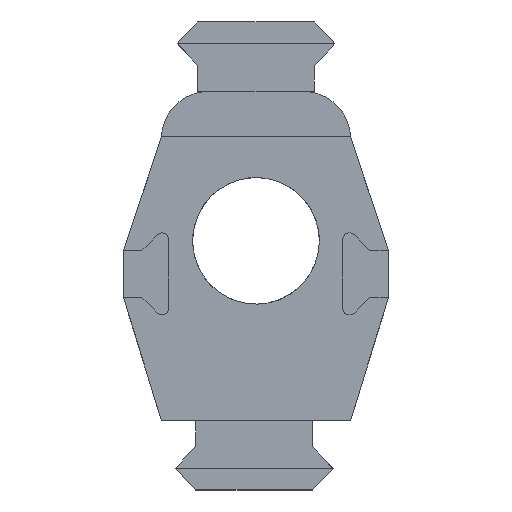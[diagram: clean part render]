
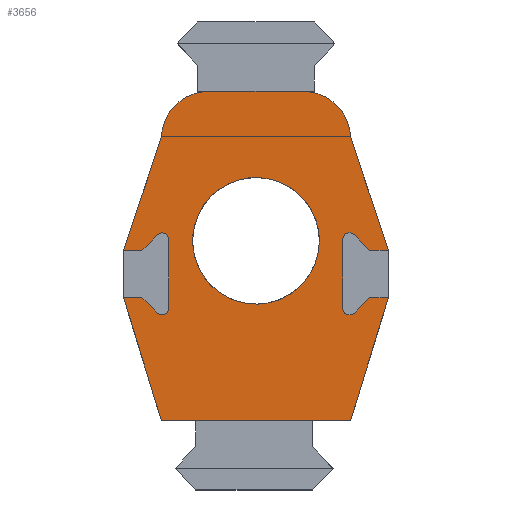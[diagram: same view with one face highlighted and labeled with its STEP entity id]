
A CAD part, front view. The second image highlights one B-rep face of the part: STEP entity #3656.
In plain terms, the highlighted planar face has unit normal (0, -1, 0).
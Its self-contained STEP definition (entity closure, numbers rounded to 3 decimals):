
#32=FACE_BOUND('',#323,.T.);
#36=ELLIPSE('',#3889,3.676,2.54);
#37=ELLIPSE('',#3892,3.676,2.54);
#56=CIRCLE('',#3868,0.889);
#58=CIRCLE('',#3872,0.889);
#60=CIRCLE('',#3878,0.889);
#62=CIRCLE('',#3882,0.889);
#64=CIRCLE('',#3890,6.35);
#65=CIRCLE('',#3891,6.35);
#66=CIRCLE('',#3893,8.5);
#67=CIRCLE('',#3894,8.5);
#117=FACE_OUTER_BOUND('',#322,.T.);
#322=EDGE_LOOP('',(#2455,#2456,#2457,#2458,#2459,#2460,#2461,#2462,#2463,
#2464,#2465,#2466,#2467,#2468,#2469,#2470,#2471,#2472,#2473,#2474,#2475,
#2476,#2477,#2478));
#323=EDGE_LOOP('',(#2479,#2480));
#515=LINE('',#5106,#1007);
#519=LINE('',#5115,#1011);
#523=LINE('',#5123,#1015);
#527=LINE('',#5135,#1019);
#531=LINE('',#5146,#1023);
#534=LINE('',#5153,#1026);
#539=LINE('',#5167,#1031);
#543=LINE('',#5179,#1035);
#546=LINE('',#5185,#1038);
#549=LINE('',#5191,#1041);
#554=LINE('',#5203,#1046);
#555=LINE('',#5205,#1047);
#556=LINE('',#5209,#1048);
#557=LINE('',#5212,#1049);
#558=LINE('',#5214,#1050);
#559=LINE('',#5217,#1051);
#1007=VECTOR('',#4116,10.);
#1011=VECTOR('',#4122,10.);
#1015=VECTOR('',#4128,10.);
#1019=VECTOR('',#4140,10.);
#1023=VECTOR('',#4152,10.);
#1026=VECTOR('',#4159,10.);
#1031=VECTOR('',#4172,10.);
#1035=VECTOR('',#4184,10.);
#1038=VECTOR('',#4189,10.);
#1041=VECTOR('',#4194,10.);
#1046=VECTOR('',#4205,10.);
#1047=VECTOR('',#4206,10.);
#1048=VECTOR('',#4209,10.);
#1049=VECTOR('',#4212,10.);
#1050=VECTOR('',#4213,10.);
#1051=VECTOR('',#4216,10.);
#1499=VERTEX_POINT('',#5104);
#1500=VERTEX_POINT('',#5105);
#1503=VERTEX_POINT('',#5113);
#1504=VERTEX_POINT('',#5114);
#1507=VERTEX_POINT('',#5122);
#1509=VERTEX_POINT('',#5128);
#1511=VERTEX_POINT('',#5134);
#1513=VERTEX_POINT('',#5140);
#1515=VERTEX_POINT('',#5151);
#1516=VERTEX_POINT('',#5152);
#1519=VERTEX_POINT('',#5160);
#1521=VERTEX_POINT('',#5166);
#1523=VERTEX_POINT('',#5172);
#1525=VERTEX_POINT('',#5178);
#1527=VERTEX_POINT('',#5184);
#1529=VERTEX_POINT('',#5190);
#1532=VERTEX_POINT('',#5200);
#1533=VERTEX_POINT('',#5201);
#1534=VERTEX_POINT('',#5204);
#1535=VERTEX_POINT('',#5206);
#1536=VERTEX_POINT('',#5208);
#1537=VERTEX_POINT('',#5210);
#1538=VERTEX_POINT('',#5213);
#1539=VERTEX_POINT('',#5215);
#1540=VERTEX_POINT('',#5218);
#1541=VERTEX_POINT('',#5219);
#1843=EDGE_CURVE('',#1499,#1500,#515,.T.);
#1847=EDGE_CURVE('',#1503,#1504,#519,.T.);
#1851=EDGE_CURVE('',#1500,#1507,#523,.T.);
#1854=EDGE_CURVE('',#1507,#1509,#56,.T.);
#1857=EDGE_CURVE('',#1509,#1511,#527,.T.);
#1860=EDGE_CURVE('',#1511,#1513,#58,.T.);
#1863=EDGE_CURVE('',#1513,#1503,#531,.T.);
#1866=EDGE_CURVE('',#1515,#1516,#534,.T.);
#1870=EDGE_CURVE('',#1519,#1515,#60,.T.);
#1873=EDGE_CURVE('',#1521,#1519,#539,.T.);
#1876=EDGE_CURVE('',#1523,#1521,#62,.T.);
#1879=EDGE_CURVE('',#1525,#1523,#543,.T.);
#1882=EDGE_CURVE('',#1516,#1527,#546,.T.);
#1885=EDGE_CURVE('',#1529,#1525,#549,.T.);
#1890=EDGE_CURVE('',#1532,#1533,#36,.T.);
#1891=EDGE_CURVE('',#1533,#1499,#554,.T.);
#1892=EDGE_CURVE('',#1504,#1534,#555,.T.);
#1893=EDGE_CURVE('',#1534,#1535,#64,.T.);
#1894=EDGE_CURVE('',#1535,#1536,#556,.T.);
#1895=EDGE_CURVE('',#1536,#1537,#65,.T.);
#1896=EDGE_CURVE('',#1537,#1529,#557,.T.);
#1897=EDGE_CURVE('',#1527,#1538,#558,.T.);
#1898=EDGE_CURVE('',#1538,#1539,#37,.T.);
#1899=EDGE_CURVE('',#1539,#1532,#559,.T.);
#1900=EDGE_CURVE('',#1540,#1541,#66,.T.);
#1901=EDGE_CURVE('',#1541,#1540,#67,.T.);
#2455=ORIENTED_EDGE('',*,*,#1890,.T.);
#2456=ORIENTED_EDGE('',*,*,#1891,.T.);
#2457=ORIENTED_EDGE('',*,*,#1843,.T.);
#2458=ORIENTED_EDGE('',*,*,#1851,.T.);
#2459=ORIENTED_EDGE('',*,*,#1854,.T.);
#2460=ORIENTED_EDGE('',*,*,#1857,.T.);
#2461=ORIENTED_EDGE('',*,*,#1860,.T.);
#2462=ORIENTED_EDGE('',*,*,#1863,.T.);
#2463=ORIENTED_EDGE('',*,*,#1847,.T.);
#2464=ORIENTED_EDGE('',*,*,#1892,.T.);
#2465=ORIENTED_EDGE('',*,*,#1893,.T.);
#2466=ORIENTED_EDGE('',*,*,#1894,.T.);
#2467=ORIENTED_EDGE('',*,*,#1895,.T.);
#2468=ORIENTED_EDGE('',*,*,#1896,.T.);
#2469=ORIENTED_EDGE('',*,*,#1885,.T.);
#2470=ORIENTED_EDGE('',*,*,#1879,.T.);
#2471=ORIENTED_EDGE('',*,*,#1876,.T.);
#2472=ORIENTED_EDGE('',*,*,#1873,.T.);
#2473=ORIENTED_EDGE('',*,*,#1870,.T.);
#2474=ORIENTED_EDGE('',*,*,#1866,.T.);
#2475=ORIENTED_EDGE('',*,*,#1882,.T.);
#2476=ORIENTED_EDGE('',*,*,#1897,.T.);
#2477=ORIENTED_EDGE('',*,*,#1898,.T.);
#2478=ORIENTED_EDGE('',*,*,#1899,.T.);
#2479=ORIENTED_EDGE('',*,*,#1900,.T.);
#2480=ORIENTED_EDGE('',*,*,#1901,.T.);
#3472=PLANE('',#3888);
#3656=ADVANCED_FACE('',(#117,#32),#3472,.F.);
#3868=AXIS2_PLACEMENT_3D('',#5129,#4133,#4134);
#3872=AXIS2_PLACEMENT_3D('',#5141,#4145,#4146);
#3878=AXIS2_PLACEMENT_3D('',#5161,#4165,#4166);
#3882=AXIS2_PLACEMENT_3D('',#5173,#4177,#4178);
#3888=AXIS2_PLACEMENT_3D('',#5199,#4201,#4202);
#3889=AXIS2_PLACEMENT_3D('',#5202,#4203,#4204);
#3890=AXIS2_PLACEMENT_3D('',#5207,#4207,#4208);
#3891=AXIS2_PLACEMENT_3D('',#5211,#4210,#4211);
#3892=AXIS2_PLACEMENT_3D('',#5216,#4214,#4215);
#3893=AXIS2_PLACEMENT_3D('',#5220,#4217,#4218);
#3894=AXIS2_PLACEMENT_3D('',#5221,#4219,#4220);
#4116=DIRECTION('',(-1.,0.,0.));
#4122=DIRECTION('',(1.,0.,-0.001));
#4128=DIRECTION('',(-0.707,0.,-0.707));
#4133=DIRECTION('center_axis',(0.,1.,0.));
#4134=DIRECTION('ref_axis',(0.707,0.,-0.707));
#4140=DIRECTION('',(0.,0.,1.));
#4145=DIRECTION('center_axis',(0.,1.,0.));
#4146=DIRECTION('ref_axis',(-1.,0.,0.));
#4152=DIRECTION('',(0.707,0.,-0.707));
#4159=DIRECTION('',(-0.707,0.,0.707));
#4165=DIRECTION('center_axis',(0.,1.,0.));
#4166=DIRECTION('ref_axis',(1.,0.,0.));
#4172=DIRECTION('',(0.,0.,-1.));
#4177=DIRECTION('center_axis',(0.,1.,0.));
#4178=DIRECTION('ref_axis',(-0.707,0.,0.707));
#4184=DIRECTION('',(0.707,0.,0.707));
#4189=DIRECTION('',(-1.,0.,0.));
#4194=DIRECTION('',(1.,0.,0.001));
#4201=DIRECTION('center_axis',(0.,1.,0.));
#4202=DIRECTION('ref_axis',(-1.,0.,0.));
#4203=DIRECTION('center_axis',(0.,-1.,0.));
#4204=DIRECTION('ref_axis',(-0.294,0.,-0.956));
#4205=DIRECTION('',(0.294,0.,0.956));
#4206=DIRECTION('',(-0.316,0.,0.949));
#4207=DIRECTION('center_axis',(0.,-1.,0.));
#4208=DIRECTION('ref_axis',(0.999,0.,0.04));
#4209=DIRECTION('',(-1.,0.,0.));
#4210=DIRECTION('center_axis',(0.,-1.,0.));
#4211=DIRECTION('ref_axis',(-0.999,0.,0.04));
#4212=DIRECTION('',(-0.316,0.,-0.949));
#4213=DIRECTION('',(0.294,0.,-0.956));
#4214=DIRECTION('center_axis',(0.,-1.,0.));
#4215=DIRECTION('ref_axis',(0.294,0.,-0.956));
#4216=DIRECTION('',(1.,0.,0.));
#4217=DIRECTION('center_axis',(0.,1.,0.));
#4218=DIRECTION('ref_axis',(-1.,0.,0.));
#4219=DIRECTION('center_axis',(0.,1.,0.));
#4220=DIRECTION('ref_axis',(-1.,0.,0.));
#5104=CARTESIAN_POINT('',(17.78,171.04,3.81));
#5105=CARTESIAN_POINT('',(15.24,171.04,3.81));
#5106=CARTESIAN_POINT('',(8.89,171.04,3.81));
#5113=CARTESIAN_POINT('',(15.24,171.04,10.163));
#5114=CARTESIAN_POINT('',(17.78,171.04,10.16));
#5115=CARTESIAN_POINT('',(7.622,171.04,10.172));
#5122=CARTESIAN_POINT('',(13.166,171.04,1.736));
#5123=CARTESIAN_POINT('',(12.065,171.04,0.635));
#5128=CARTESIAN_POINT('',(11.648,171.04,2.364));
#5129=CARTESIAN_POINT('Origin',(12.537,171.04,2.364));
#5134=CARTESIAN_POINT('',(11.648,171.04,11.609));
#5135=CARTESIAN_POINT('',(11.648,171.04,4.357));
#5140=CARTESIAN_POINT('',(13.166,171.04,12.238));
#5141=CARTESIAN_POINT('Origin',(12.537,171.04,11.609));
#5146=CARTESIAN_POINT('',(11.346,171.04,14.057));
#5151=CARTESIAN_POINT('',(-13.243,171.04,1.736));
#5152=CARTESIAN_POINT('',(-15.317,171.04,3.81));
#5153=CARTESIAN_POINT('',(-11.086,171.04,-0.422));
#5160=CARTESIAN_POINT('',(-11.725,171.04,2.364));
#5161=CARTESIAN_POINT('Origin',(-12.614,171.04,2.364));
#5166=CARTESIAN_POINT('',(-11.725,171.04,11.609));
#5167=CARTESIAN_POINT('',(-11.725,171.04,8.979));
#5172=CARTESIAN_POINT('',(-13.243,171.04,12.238));
#5173=CARTESIAN_POINT('Origin',(-12.614,171.04,11.609));
#5178=CARTESIAN_POINT('',(-15.317,171.04,10.163));
#5179=CARTESIAN_POINT('',(-12.441,171.04,13.039));
#5184=CARTESIAN_POINT('',(-17.78,171.04,3.81));
#5185=CARTESIAN_POINT('',(-7.659,171.04,3.81));
#5190=CARTESIAN_POINT('',(-17.78,171.04,10.16));
#5191=CARTESIAN_POINT('',(-8.892,171.04,10.171));
#5199=CARTESIAN_POINT('Origin',(0.,171.04,6.35));
#5200=CARTESIAN_POINT('',(12.69,171.04,-12.699));
#5201=CARTESIAN_POINT('',(12.794,171.04,-12.394));
#5202=CARTESIAN_POINT('Origin',(10.366,171.04,-11.647));
#5203=CARTESIAN_POINT('',(17.368,171.04,2.471));
#5204=CARTESIAN_POINT('',(12.7,171.04,25.4));
#5205=CARTESIAN_POINT('',(14.923,171.04,18.733));
#5206=CARTESIAN_POINT('',(6.355,171.04,31.496));
#5207=CARTESIAN_POINT('Origin',(6.355,171.04,25.146));
#5208=CARTESIAN_POINT('',(-6.355,171.04,31.496));
#5209=CARTESIAN_POINT('',(-6.35,171.04,31.496));
#5210=CARTESIAN_POINT('',(-12.7,171.04,25.4));
#5211=CARTESIAN_POINT('Origin',(-6.355,171.04,25.146));
#5212=CARTESIAN_POINT('',(-17.463,171.04,11.113));
#5213=CARTESIAN_POINT('',(-12.794,171.04,-12.394));
#5214=CARTESIAN_POINT('',(-14.828,171.04,-5.784));
#5215=CARTESIAN_POINT('',(-12.69,171.04,-12.699));
#5216=CARTESIAN_POINT('Origin',(-10.366,171.04,-11.647));
#5217=CARTESIAN_POINT('',(6.35,171.04,-12.699));
#5218=CARTESIAN_POINT('',(8.064,171.04,14.118));
#5219=CARTESIAN_POINT('',(8.5,171.04,11.43));
#5220=CARTESIAN_POINT('Origin',(0.,171.04,11.43));
#5221=CARTESIAN_POINT('Origin',(0.,171.04,11.43));
